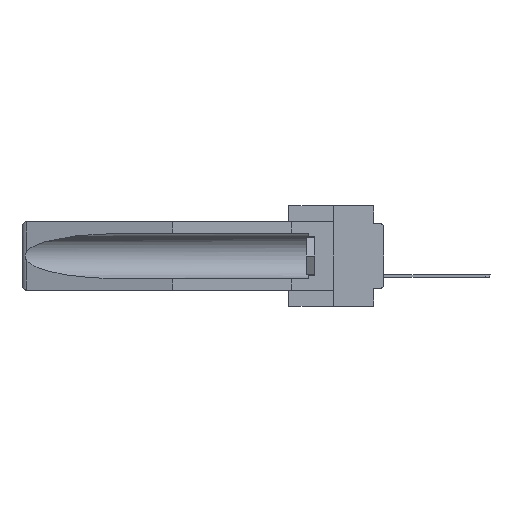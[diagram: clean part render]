
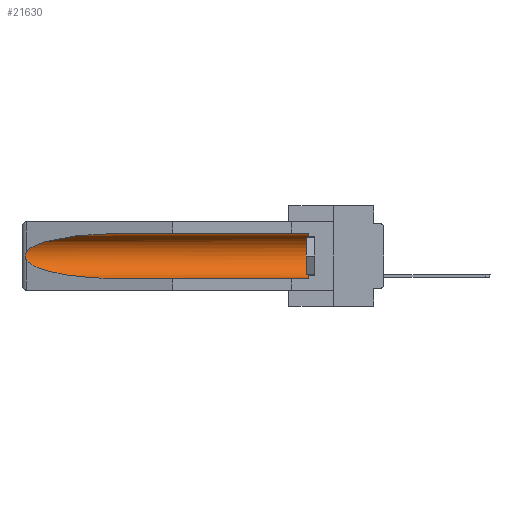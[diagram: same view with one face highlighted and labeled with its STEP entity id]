
A CAD part, left-side view. The second image highlights one B-rep face of the part: STEP entity #21630.
In plain terms, the highlighted cylindrical face has radius 2.857 mm (diameter 5.715 mm), a partial arc.
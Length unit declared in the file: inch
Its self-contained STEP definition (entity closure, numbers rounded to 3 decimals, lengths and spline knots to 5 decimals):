
#30 = ORIENTED_EDGE ( 'NONE', *, *, #11834, .T. ) ;
#461 = DIRECTION ( 'NONE',  ( 0., 1., 0. ) ) ;
#1893 = CARTESIAN_POINT ( 'NONE',  ( 0.26537, 1.52718, -0.14972 ) ) ;
#2514 = CARTESIAN_POINT ( 'NONE',  ( 0.155, 0.126, -0.1715 ) ) ;
#3488 = B_SPLINE_CURVE_WITH_KNOTS ( 'NONE', 3,
 ( #7776, #25916, #18128, #25907, #5599, #19646, #14152, #28816, #5843, #32640 ),
 .UNSPECIFIED., .F., .F.,
 ( 4, 2, 2, 2, 4 ),
 ( 0., 0.00029, 0.00058, 0.00087, 0.00117 ),
 .UNSPECIFIED. ) ;
#5577 = CARTESIAN_POINT ( 'NONE',  ( 0.155, 0.126, -0.059 ) ) ;
#5599 = CARTESIAN_POINT ( 'NONE',  ( 0.2675, 1.53308, -0.16763 ) ) ;
#5688 = EDGE_CURVE ( 'NONE', #7830, #10445, #12048, .T. ) ;
#5843 = CARTESIAN_POINT ( 'NONE',  ( 0.26597, 1.5296, -0.19026 ) ) ;
#6222 = VERTEX_POINT ( 'NONE', #22093 ) ;
#7776 = CARTESIAN_POINT ( 'NONE',  ( 0.26537, 1.52718, -0.14972 ) ) ;
#7830 = VERTEX_POINT ( 'NONE', #25069 ) ;
#9305 = VERTEX_POINT ( 'NONE', #13076 ) ;
#9812 = ORIENTED_EDGE ( 'NONE', *, *, #15811, .T. ) ;
#10052 = CARTESIAN_POINT ( 'NONE',  ( 0.155, 1.07973, -0.284 ) ) ;
#10445 = VERTEX_POINT ( 'NONE', #5577 ) ;
#10861 = ORIENTED_EDGE ( 'NONE', *, *, #19777, .T. ) ;
#11834 = EDGE_CURVE ( 'NONE', #19497, #32915, #16464, .T. ) ;
#12048 = CIRCLE ( 'NONE', #19989, 0.1125 ) ;
#12541 = VECTOR ( 'NONE', #18912, 39.37008 ) ;
#12634 = CARTESIAN_POINT ( 'NONE',  ( 0.26537, 1.52718, -0.19328 ) ) ;
#12658 = ORIENTED_EDGE ( 'NONE', *, *, #32464, .T. ) ;
#13076 = CARTESIAN_POINT ( 'NONE',  ( 0.26537, 1.52718, -0.19328 ) ) ;
#14152 = CARTESIAN_POINT ( 'NONE',  ( 0.2673, 1.53269, -0.17917 ) ) ;
#14980 = CARTESIAN_POINT ( 'NONE',  ( 0.21114, 1.30732, -0.059 ) ) ;
#15811 = EDGE_CURVE ( 'NONE', #32915, #9305, #3488, .T. ) ;
#16326 = CARTESIAN_POINT ( 'NONE',  ( 0.155, -0.30754, -0.059 ) ) ;
#16464 =( BOUNDED_CURVE ( )  B_SPLINE_CURVE ( 3, ( #30279, #14980, #32832, #1893 ),
 .UNSPECIFIED., .F., .F. ) 
 B_SPLINE_CURVE_WITH_KNOTS ( ( 4, 4 ),
 ( 4.71239, 6.08839 ),
 .UNSPECIFIED. ) 
 CURVE ( )  GEOMETRIC_REPRESENTATION_ITEM ( )  RATIONAL_B_SPLINE_CURVE ( ( 1., 0.848, 0.848, 1. ) ) 
 REPRESENTATION_ITEM ( '' )  );
#17383 = CARTESIAN_POINT ( 'NONE',  ( 0.26537, 1.52718, -0.14972 ) ) ;
#17573 = EDGE_LOOP ( 'NONE', ( #30, #9812, #10861, #20773, #30038, #12658 ) ) ;
#18128 = CARTESIAN_POINT ( 'NONE',  ( 0.26654, 1.53092, -0.15636 ) ) ;
#18879 = LINE ( 'NONE', #21781, #22432 ) ;
#18912 = DIRECTION ( 'NONE',  ( 0., 1., 0. ) ) ;
#18936 = CYLINDRICAL_SURFACE ( 'NONE', #29541, 0.1125 ) ;
#19497 = VERTEX_POINT ( 'NONE', #31698 ) ;
#19646 = CARTESIAN_POINT ( 'NONE',  ( 0.2675, 1.53308, -0.17534 ) ) ;
#19777 = EDGE_CURVE ( 'NONE', #9305, #6222, #30825, .T. ) ;
#19989 = AXIS2_PLACEMENT_3D ( 'NONE', #2514, #30556, #20488 ) ;
#20187 = DIRECTION ( 'NONE',  ( 0., 1., 0. ) ) ;
#20488 = DIRECTION ( 'NONE',  ( 0., 0., 1. ) ) ;
#20773 = ORIENTED_EDGE ( 'NONE', *, *, #26688, .F. ) ;
#21630 = ADVANCED_FACE ( 'NONE', ( #22147 ), #18936, .F. ) ;
#21781 = CARTESIAN_POINT ( 'NONE',  ( 0.155, -0.30754, -0.284 ) ) ;
#22093 = CARTESIAN_POINT ( 'NONE',  ( 0.155, 1.07973, -0.284 ) ) ;
#22147 = FACE_OUTER_BOUND ( 'NONE', #17573, .T. ) ;
#22432 = VECTOR ( 'NONE', #461, 39.37008 ) ;
#24946 = CARTESIAN_POINT ( 'NONE',  ( 0.21114, 1.30732, -0.284 ) ) ;
#25002 = CARTESIAN_POINT ( 'NONE',  ( 0.155, -0.30754, -0.1715 ) ) ;
#25069 = CARTESIAN_POINT ( 'NONE',  ( 0.155, 0.126, -0.284 ) ) ;
#25665 = DIRECTION ( 'NONE',  ( 0., 0., 1. ) ) ;
#25907 = CARTESIAN_POINT ( 'NONE',  ( 0.2673, 1.5327, -0.16383 ) ) ;
#25916 = CARTESIAN_POINT ( 'NONE',  ( 0.26597, 1.52961, -0.15275 ) ) ;
#26688 = EDGE_CURVE ( 'NONE', #7830, #6222, #18879, .T. ) ;
#27766 = LINE ( 'NONE', #16326, #12541 ) ;
#28816 = CARTESIAN_POINT ( 'NONE',  ( 0.26655, 1.53094, -0.18657 ) ) ;
#29541 = AXIS2_PLACEMENT_3D ( 'NONE', #25002, #20187, #25665 ) ;
#30038 = ORIENTED_EDGE ( 'NONE', *, *, #5688, .T. ) ;
#30279 = CARTESIAN_POINT ( 'NONE',  ( 0.155, 1.07973, -0.059 ) ) ;
#30556 = DIRECTION ( 'NONE',  ( 0., -1., 0. ) ) ;
#30825 =( BOUNDED_CURVE ( )  B_SPLINE_CURVE ( 3, ( #12634, #32650, #24946, #10052 ),
 .UNSPECIFIED., .F., .F. ) 
 B_SPLINE_CURVE_WITH_KNOTS ( ( 4, 4 ),
 ( 0.1948, 1.5708 ),
 .UNSPECIFIED. ) 
 CURVE ( )  GEOMETRIC_REPRESENTATION_ITEM ( )  RATIONAL_B_SPLINE_CURVE ( ( 1., 0.848, 0.848, 1. ) ) 
 REPRESENTATION_ITEM ( '' )  );
#31698 = CARTESIAN_POINT ( 'NONE',  ( 0.155, 1.07973, -0.059 ) ) ;
#32464 = EDGE_CURVE ( 'NONE', #10445, #19497, #27766, .T. ) ;
#32640 = CARTESIAN_POINT ( 'NONE',  ( 0.26537, 1.52718, -0.19328 ) ) ;
#32650 = CARTESIAN_POINT ( 'NONE',  ( 0.25451, 1.48313, -0.24835 ) ) ;
#32832 = CARTESIAN_POINT ( 'NONE',  ( 0.25451, 1.48313, -0.09465 ) ) ;
#32915 = VERTEX_POINT ( 'NONE', #17383 ) ;
